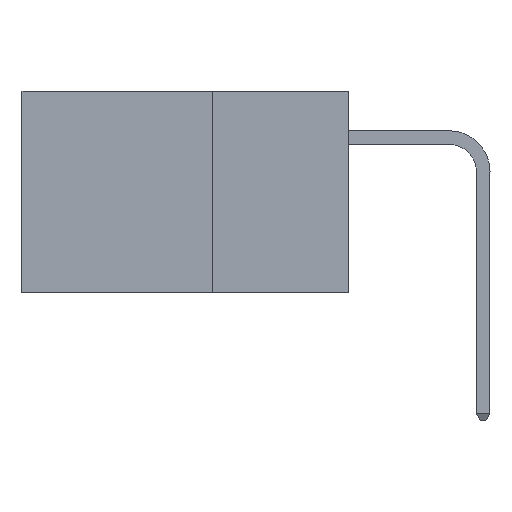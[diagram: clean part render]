
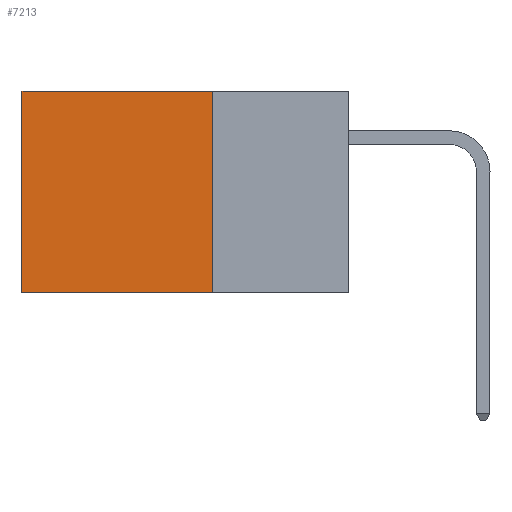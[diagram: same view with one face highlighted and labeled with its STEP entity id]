
A CAD part, left-side view. The second image highlights one B-rep face of the part: STEP entity #7213.
In plain terms, the highlighted planar face has unit normal (-1, 0, 0).
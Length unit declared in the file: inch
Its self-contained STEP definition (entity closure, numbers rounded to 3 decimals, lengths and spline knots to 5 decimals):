
#677 = DIRECTION ( 'NONE',  ( 1., 0., 0. ) ) ;
#2463 = VECTOR ( 'NONE', #4653, 39.37008 ) ;
#2774 = CARTESIAN_POINT ( 'NONE',  ( 0.2875, 0.25, 0. ) ) ;
#4372 = ORIENTED_EDGE ( 'NONE', *, *, #23119, .F. ) ;
#4653 = DIRECTION ( 'NONE',  ( 0., 1., 0. ) ) ;
#4859 = LINE ( 'NONE', #12034, #13707 ) ;
#4974 = CARTESIAN_POINT ( 'NONE',  ( 0.2875, 0.6, 0. ) ) ;
#6178 = EDGE_CURVE ( 'NONE', #16014, #10826, #16026, .T. ) ;
#6254 = LINE ( 'NONE', #12681, #2463 ) ;
#6519 = ORIENTED_EDGE ( 'NONE', *, *, #6178, .T. ) ;
#7211 = DIRECTION ( 'NONE',  ( 0., 0., -1. ) ) ;
#7213 = ADVANCED_FACE ( 'NONE', ( #9908 ), #16822, .F. ) ;
#8037 = CARTESIAN_POINT ( 'NONE',  ( 0.2875, 0.25, 0. ) ) ;
#8541 = DIRECTION ( 'NONE',  ( 0., 0., -1. ) ) ;
#8922 = AXIS2_PLACEMENT_3D ( 'NONE', #2774, #677, #8541 ) ;
#8936 = LINE ( 'NONE', #22879, #9792 ) ;
#9542 = ORIENTED_EDGE ( 'NONE', *, *, #14161, .F. ) ;
#9792 = VECTOR ( 'NONE', #7211, 39.37008 ) ;
#9908 = FACE_OUTER_BOUND ( 'NONE', #18347, .T. ) ;
#10826 = VERTEX_POINT ( 'NONE', #4974 ) ;
#12034 = CARTESIAN_POINT ( 'NONE',  ( 0.2875, 0.6, 0. ) ) ;
#12681 = CARTESIAN_POINT ( 'NONE',  ( 0.2875, 0.25, -0.37 ) ) ;
#12754 = CARTESIAN_POINT ( 'NONE',  ( 0.2875, 0.25, -0.37 ) ) ;
#13175 = CARTESIAN_POINT ( 'NONE',  ( 0.2875, 0.25, 0. ) ) ;
#13182 = CARTESIAN_POINT ( 'NONE',  ( 0.2875, 0.6, -0.37 ) ) ;
#13366 = EDGE_CURVE ( 'NONE', #10826, #23620, #4859, .T. ) ;
#13707 = VECTOR ( 'NONE', #16121, 39.37008 ) ;
#14161 = EDGE_CURVE ( 'NONE', #16014, #17199, #8936, .T. ) ;
#16014 = VERTEX_POINT ( 'NONE', #13175 ) ;
#16026 = LINE ( 'NONE', #8037, #18872 ) ;
#16121 = DIRECTION ( 'NONE',  ( 0., 0., -1. ) ) ;
#16822 = PLANE ( 'NONE',  #8922 ) ;
#17055 = ORIENTED_EDGE ( 'NONE', *, *, #13366, .T. ) ;
#17199 = VERTEX_POINT ( 'NONE', #12754 ) ;
#18347 = EDGE_LOOP ( 'NONE', ( #17055, #4372, #9542, #6519 ) ) ;
#18872 = VECTOR ( 'NONE', #20332, 39.37008 ) ;
#20332 = DIRECTION ( 'NONE',  ( 0., 1., 0. ) ) ;
#22879 = CARTESIAN_POINT ( 'NONE',  ( 0.2875, 0.25, 0. ) ) ;
#23119 = EDGE_CURVE ( 'NONE', #17199, #23620, #6254, .T. ) ;
#23620 = VERTEX_POINT ( 'NONE', #13182 ) ;
